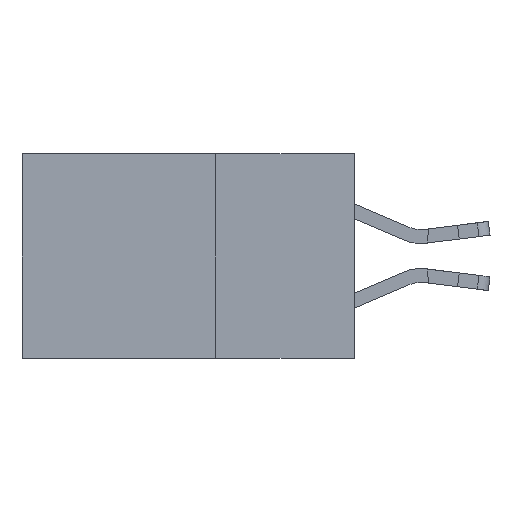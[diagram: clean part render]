
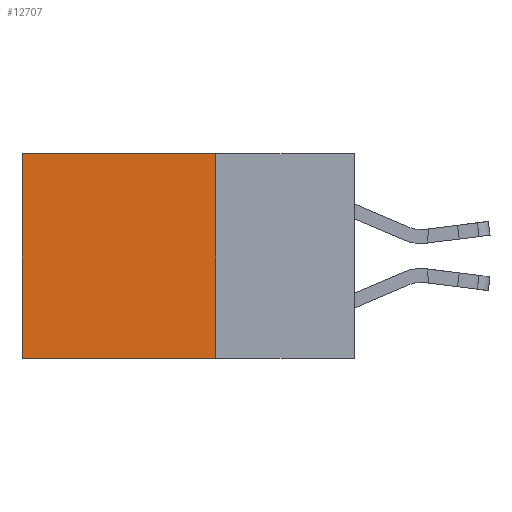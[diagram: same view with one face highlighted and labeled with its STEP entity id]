
A CAD part, left-side view. The second image highlights one B-rep face of the part: STEP entity #12707.
In plain terms, the highlighted planar face has unit normal (-1, 0, 0).
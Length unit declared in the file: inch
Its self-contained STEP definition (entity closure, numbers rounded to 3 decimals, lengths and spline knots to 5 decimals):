
#96 = EDGE_CURVE ( 'NONE', #12753, #7367, #13317, .T. ) ;
#982 = PLANE ( 'NONE',  #5628 ) ;
#1246 = LINE ( 'NONE', #2474, #1962 ) ;
#1578 = DIRECTION ( 'NONE',  ( 0., 1., 0. ) ) ;
#1734 = CARTESIAN_POINT ( 'NONE',  ( 0.2615, 0.6, 0. ) ) ;
#1810 = EDGE_CURVE ( 'NONE', #12753, #3784, #7047, .T. ) ;
#1962 = VECTOR ( 'NONE', #11904, 39.37008 ) ;
#2059 = FACE_OUTER_BOUND ( 'NONE', #4165, .T. ) ;
#2275 = DIRECTION ( 'NONE',  ( 1., 0., 0. ) ) ;
#2294 = CARTESIAN_POINT ( 'NONE',  ( 0.2615, 0.25, -0.37 ) ) ;
#2474 = CARTESIAN_POINT ( 'NONE',  ( 0.2615, 0.25, -0.37 ) ) ;
#2527 = EDGE_CURVE ( 'NONE', #3784, #13180, #8194, .T. ) ;
#2821 = VECTOR ( 'NONE', #12517, 39.37008 ) ;
#2974 = ORIENTED_EDGE ( 'NONE', *, *, #96, .F. ) ;
#3323 = VECTOR ( 'NONE', #7216, 39.37008 ) ;
#3784 = VERTEX_POINT ( 'NONE', #1734 ) ;
#3872 = CARTESIAN_POINT ( 'NONE',  ( 0.2615, 0.6, -0.37 ) ) ;
#4165 = EDGE_LOOP ( 'NONE', ( #7055, #5668, #2974, #13979 ) ) ;
#5602 = DIRECTION ( 'NONE',  ( 0., 0., -1. ) ) ;
#5628 = AXIS2_PLACEMENT_3D ( 'NONE', #8657, #2275, #5602 ) ;
#5668 = ORIENTED_EDGE ( 'NONE', *, *, #5858, .F. ) ;
#5674 = CARTESIAN_POINT ( 'NONE',  ( 0.2615, 0.25, 0. ) ) ;
#5858 = EDGE_CURVE ( 'NONE', #7367, #13180, #1246, .T. ) ;
#5984 = VECTOR ( 'NONE', #1578, 39.37008 ) ;
#7047 = LINE ( 'NONE', #12287, #5984 ) ;
#7055 = ORIENTED_EDGE ( 'NONE', *, *, #2527, .T. ) ;
#7216 = DIRECTION ( 'NONE',  ( 0., 0., -1. ) ) ;
#7367 = VERTEX_POINT ( 'NONE', #2294 ) ;
#8194 = LINE ( 'NONE', #3872, #2821 ) ;
#8277 = CARTESIAN_POINT ( 'NONE',  ( 0.2615, 0.25, -0.37 ) ) ;
#8574 = CARTESIAN_POINT ( 'NONE',  ( 0.2615, 0.6, -0.37 ) ) ;
#8657 = CARTESIAN_POINT ( 'NONE',  ( 0.2615, 0.25, -0.37 ) ) ;
#11904 = DIRECTION ( 'NONE',  ( 0., 1., 0. ) ) ;
#12287 = CARTESIAN_POINT ( 'NONE',  ( 0.2615, 0.25, 0. ) ) ;
#12517 = DIRECTION ( 'NONE',  ( 0., 0., -1. ) ) ;
#12707 = ADVANCED_FACE ( 'NONE', ( #2059 ), #982, .F. ) ;
#12753 = VERTEX_POINT ( 'NONE', #5674 ) ;
#13180 = VERTEX_POINT ( 'NONE', #8574 ) ;
#13317 = LINE ( 'NONE', #8277, #3323 ) ;
#13979 = ORIENTED_EDGE ( 'NONE', *, *, #1810, .T. ) ;
